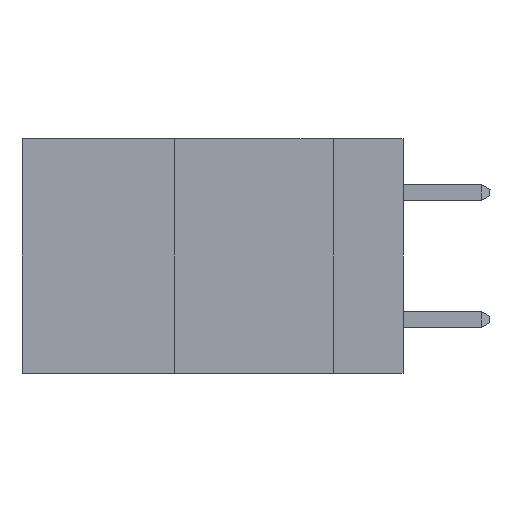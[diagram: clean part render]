
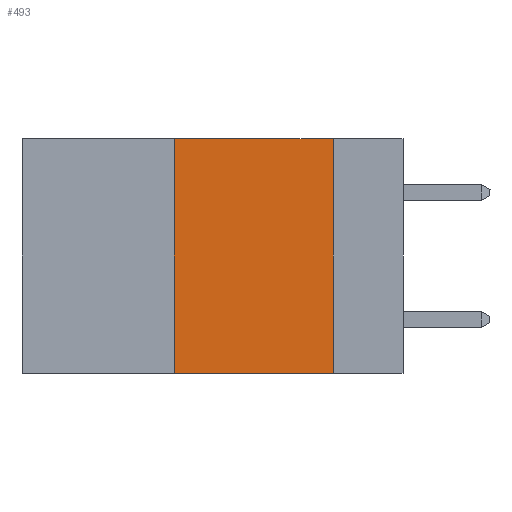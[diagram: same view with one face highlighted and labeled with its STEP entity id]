
A CAD part, left-side view. The second image highlights one B-rep face of the part: STEP entity #493.
In plain terms, the highlighted planar face has unit normal (-1, 0, 0).
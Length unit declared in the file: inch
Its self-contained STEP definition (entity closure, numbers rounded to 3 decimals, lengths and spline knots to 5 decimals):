
#176 = EDGE_CURVE ( 'NONE', #378, #7837, #15405, .T. ) ;
#228 = LINE ( 'NONE', #28130, #5110 ) ;
#378 = VERTEX_POINT ( 'NONE', #16886 ) ;
#493 = ADVANCED_FACE ( 'NONE', ( #4099 ), #1553, .F. ) ;
#1553 = PLANE ( 'NONE',  #22387 ) ;
#1582 = CARTESIAN_POINT ( 'NONE',  ( 0., 0.6, 0. ) ) ;
#1951 = VERTEX_POINT ( 'NONE', #19228 ) ;
#1977 = VECTOR ( 'NONE', #8315, 39.37008 ) ;
#4052 = CARTESIAN_POINT ( 'NONE',  ( 0., 0.36, 0. ) ) ;
#4099 = FACE_OUTER_BOUND ( 'NONE', #10855, .T. ) ;
#4105 = EDGE_CURVE ( 'NONE', #4129, #1951, #228, .T. ) ;
#4129 = VERTEX_POINT ( 'NONE', #7730 ) ;
#4171 = EDGE_CURVE ( 'NONE', #7837, #4129, #26261, .T. ) ;
#5110 = VECTOR ( 'NONE', #18930, 39.37008 ) ;
#7730 = CARTESIAN_POINT ( 'NONE',  ( 0., 0.11, 0. ) ) ;
#7837 = VERTEX_POINT ( 'NONE', #17660 ) ;
#8315 = DIRECTION ( 'NONE',  ( 0., -1., 0. ) ) ;
#8668 = VECTOR ( 'NONE', #19847, 39.37008 ) ;
#10352 = DIRECTION ( 'NONE',  ( 1., 0., 0. ) ) ;
#10398 = CARTESIAN_POINT ( 'NONE',  ( 0., 0.6, -0.37 ) ) ;
#10855 = EDGE_LOOP ( 'NONE', ( #28648, #13908, #18387, #21430 ) ) ;
#11274 = LINE ( 'NONE', #10398, #28887 ) ;
#13540 = DIRECTION ( 'NONE',  ( 0., -1., 0. ) ) ;
#13908 = ORIENTED_EDGE ( 'NONE', *, *, #4171, .F. ) ;
#14742 = EDGE_CURVE ( 'NONE', #378, #1951, #11274, .T. ) ;
#15405 = LINE ( 'NONE', #4052, #8668 ) ;
#16886 = CARTESIAN_POINT ( 'NONE',  ( 0., 0.36, -0.37 ) ) ;
#17490 = DIRECTION ( 'NONE',  ( 0., 0., -1. ) ) ;
#17660 = CARTESIAN_POINT ( 'NONE',  ( 0., 0.36, 0. ) ) ;
#18387 = ORIENTED_EDGE ( 'NONE', *, *, #176, .F. ) ;
#18930 = DIRECTION ( 'NONE',  ( 0., 0., -1. ) ) ;
#19228 = CARTESIAN_POINT ( 'NONE',  ( 0., 0.11, -0.37 ) ) ;
#19847 = DIRECTION ( 'NONE',  ( 0., 0., 1. ) ) ;
#21430 = ORIENTED_EDGE ( 'NONE', *, *, #14742, .T. ) ;
#22387 = AXIS2_PLACEMENT_3D ( 'NONE', #28695, #10352, #17490 ) ;
#26261 = LINE ( 'NONE', #1582, #1977 ) ;
#28130 = CARTESIAN_POINT ( 'NONE',  ( 0., 0.11, 0. ) ) ;
#28648 = ORIENTED_EDGE ( 'NONE', *, *, #4105, .F. ) ;
#28695 = CARTESIAN_POINT ( 'NONE',  ( 0., 0.6, 0. ) ) ;
#28887 = VECTOR ( 'NONE', #13540, 39.37008 ) ;
